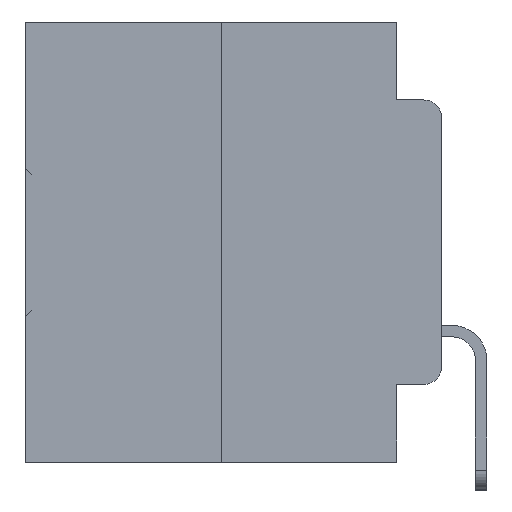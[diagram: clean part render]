
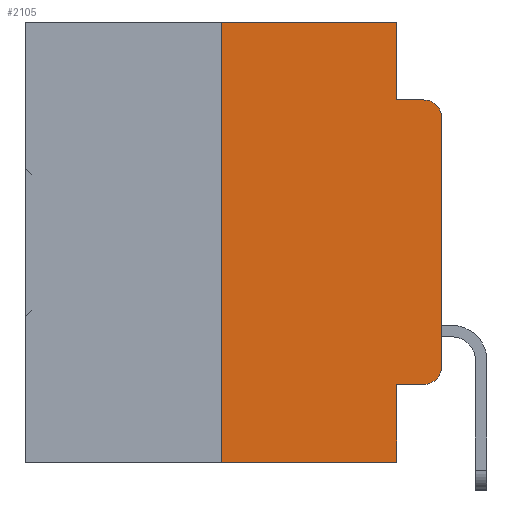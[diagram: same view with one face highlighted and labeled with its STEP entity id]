
A CAD part, left-side view. The second image highlights one B-rep face of the part: STEP entity #2105.
In plain terms, the highlighted planar face has unit normal (-1, 0, 0).
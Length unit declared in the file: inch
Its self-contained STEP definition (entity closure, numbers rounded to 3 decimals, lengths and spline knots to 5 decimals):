
#76 = DIRECTION ( 'NONE',  ( 0., 0., 1. ) ) ;
#185 = CARTESIAN_POINT ( 'NONE',  ( 0., 0.25, 0. ) ) ;
#211 = CARTESIAN_POINT ( 'NONE',  ( 0., 0.02, -0.1085 ) ) ;
#1262 = EDGE_CURVE ( 'NONE', #8069, #27537, #24713, .T. ) ;
#2105 = ADVANCED_FACE ( 'NONE', ( #28008 ), #25773, .F. ) ;
#3123 = VECTOR ( 'NONE', #12102, 39.37008 ) ;
#3181 = DIRECTION ( 'NONE',  ( 0., 0., -1. ) ) ;
#5104 = VECTOR ( 'NONE', #5820, 39.37008 ) ;
#5201 = EDGE_CURVE ( 'NONE', #32191, #29645, #11429, .T. ) ;
#5661 = CARTESIAN_POINT ( 'NONE',  ( 0., 0.051, -0.4115 ) ) ;
#5755 = VERTEX_POINT ( 'NONE', #6124 ) ;
#5820 = DIRECTION ( 'NONE',  ( 0., -1., 0. ) ) ;
#5960 = CARTESIAN_POINT ( 'NONE',  ( 0., 0.02, -0.4115 ) ) ;
#6048 = LINE ( 'NONE', #11466, #5104 ) ;
#6124 = CARTESIAN_POINT ( 'NONE',  ( 0., 0., -0.1085 ) ) ;
#6545 = CARTESIAN_POINT ( 'NONE',  ( 0., 0.051, -0.0885 ) ) ;
#6556 = CARTESIAN_POINT ( 'NONE',  ( 0., 0.051, 0. ) ) ;
#8069 = VERTEX_POINT ( 'NONE', #23046 ) ;
#8316 = LINE ( 'NONE', #30150, #22602 ) ;
#8872 = ORIENTED_EDGE ( 'NONE', *, *, #25849, .T. ) ;
#9000 = VERTEX_POINT ( 'NONE', #32117 ) ;
#9201 = EDGE_LOOP ( 'NONE', ( #27135, #14085, #15750, #16593, #31141, #31905, #26745, #13688, #29152, #8872 ) ) ;
#9254 = CARTESIAN_POINT ( 'NONE',  ( 0., 0.051, 0. ) ) ;
#9686 = AXIS2_PLACEMENT_3D ( 'NONE', #211, #19827, #3181 ) ;
#9905 = VECTOR ( 'NONE', #17113, 39.37008 ) ;
#10550 = VECTOR ( 'NONE', #25416, 39.37008 ) ;
#11006 = EDGE_CURVE ( 'NONE', #29645, #32954, #24065, .T. ) ;
#11306 = CARTESIAN_POINT ( 'NONE',  ( 0., 0.25, 0. ) ) ;
#11429 = LINE ( 'NONE', #6556, #10550 ) ;
#11466 = CARTESIAN_POINT ( 'NONE',  ( 0., 0.051, -0.4115 ) ) ;
#12102 = DIRECTION ( 'NONE',  ( 0., 0., -1. ) ) ;
#12284 = VERTEX_POINT ( 'NONE', #5661 ) ;
#13688 = ORIENTED_EDGE ( 'NONE', *, *, #34319, .F. ) ;
#14085 = ORIENTED_EDGE ( 'NONE', *, *, #14710, .T. ) ;
#14620 = DIRECTION ( 'NONE',  ( 0., -1., 0. ) ) ;
#14710 = EDGE_CURVE ( 'NONE', #5755, #32954, #21015, .T. ) ;
#14788 = DIRECTION ( 'NONE',  ( 1., 0., 0. ) ) ;
#14916 = VERTEX_POINT ( 'NONE', #20147 ) ;
#15059 = LINE ( 'NONE', #34925, #34774 ) ;
#15107 = AXIS2_PLACEMENT_3D ( 'NONE', #28344, #14788, #32848 ) ;
#15750 = ORIENTED_EDGE ( 'NONE', *, *, #11006, .F. ) ;
#15901 = DIRECTION ( 'NONE',  ( -1., 0., 0. ) ) ;
#16593 = ORIENTED_EDGE ( 'NONE', *, *, #5201, .F. ) ;
#17113 = DIRECTION ( 'NONE',  ( 0., -1., 0. ) ) ;
#18075 = EDGE_CURVE ( 'NONE', #8069, #9000, #21595, .T. ) ;
#18276 = EDGE_CURVE ( 'NONE', #14916, #5755, #15059, .T. ) ;
#19141 = CARTESIAN_POINT ( 'NONE',  ( 0., 0.02, -0.0885 ) ) ;
#19377 = AXIS2_PLACEMENT_3D ( 'NONE', #31377, #15901, #33899 ) ;
#19827 = DIRECTION ( 'NONE',  ( -1., 0., 0. ) ) ;
#20147 = CARTESIAN_POINT ( 'NONE',  ( 0., 0., -0.3915 ) ) ;
#20675 = EDGE_CURVE ( 'NONE', #27537, #32191, #8316, .T. ) ;
#21015 = CIRCLE ( 'NONE', #9686, 0.02 ) ;
#21314 = DIRECTION ( 'NONE',  ( 0., -1., 0. ) ) ;
#21595 = LINE ( 'NONE', #31535, #34386 ) ;
#22269 = VECTOR ( 'NONE', #76, 39.37008 ) ;
#22351 = CARTESIAN_POINT ( 'NONE',  ( 0., 0.051, -0.0885 ) ) ;
#22602 = VECTOR ( 'NONE', #14620, 39.37008 ) ;
#23046 = CARTESIAN_POINT ( 'NONE',  ( 0., 0.25, -0.5 ) ) ;
#24065 = LINE ( 'NONE', #22351, #9905 ) ;
#24713 = LINE ( 'NONE', #185, #22269 ) ;
#24952 = LINE ( 'NONE', #9254, #3123 ) ;
#25416 = DIRECTION ( 'NONE',  ( 0., 0., -1. ) ) ;
#25572 = CARTESIAN_POINT ( 'NONE',  ( 0., 0.051, 0. ) ) ;
#25773 = PLANE ( 'NONE',  #15107 ) ;
#25849 = EDGE_CURVE ( 'NONE', #26936, #14916, #32389, .T. ) ;
#26745 = ORIENTED_EDGE ( 'NONE', *, *, #18075, .T. ) ;
#26936 = VERTEX_POINT ( 'NONE', #5960 ) ;
#27135 = ORIENTED_EDGE ( 'NONE', *, *, #18276, .T. ) ;
#27537 = VERTEX_POINT ( 'NONE', #11306 ) ;
#28008 = FACE_OUTER_BOUND ( 'NONE', #9201, .T. ) ;
#28344 = CARTESIAN_POINT ( 'NONE',  ( 0., 0.473, 0. ) ) ;
#29152 = ORIENTED_EDGE ( 'NONE', *, *, #32643, .T. ) ;
#29645 = VERTEX_POINT ( 'NONE', #6545 ) ;
#29858 = DIRECTION ( 'NONE',  ( 0., 0., 1. ) ) ;
#30150 = CARTESIAN_POINT ( 'NONE',  ( 0., 0.473, 0. ) ) ;
#31141 = ORIENTED_EDGE ( 'NONE', *, *, #20675, .F. ) ;
#31377 = CARTESIAN_POINT ( 'NONE',  ( 0., 0.02, -0.3915 ) ) ;
#31535 = CARTESIAN_POINT ( 'NONE',  ( 0., 0.473, -0.5 ) ) ;
#31905 = ORIENTED_EDGE ( 'NONE', *, *, #1262, .F. ) ;
#32117 = CARTESIAN_POINT ( 'NONE',  ( 0., 0.051, -0.5 ) ) ;
#32191 = VERTEX_POINT ( 'NONE', #25572 ) ;
#32389 = CIRCLE ( 'NONE', #19377, 0.02 ) ;
#32643 = EDGE_CURVE ( 'NONE', #12284, #26936, #6048, .T. ) ;
#32848 = DIRECTION ( 'NONE',  ( 0., 0., -1. ) ) ;
#32954 = VERTEX_POINT ( 'NONE', #19141 ) ;
#33899 = DIRECTION ( 'NONE',  ( 0., 0., -1. ) ) ;
#34319 = EDGE_CURVE ( 'NONE', #12284, #9000, #24952, .T. ) ;
#34386 = VECTOR ( 'NONE', #21314, 39.37008 ) ;
#34774 = VECTOR ( 'NONE', #29858, 39.37008 ) ;
#34925 = CARTESIAN_POINT ( 'NONE',  ( 0., 0., 0. ) ) ;
